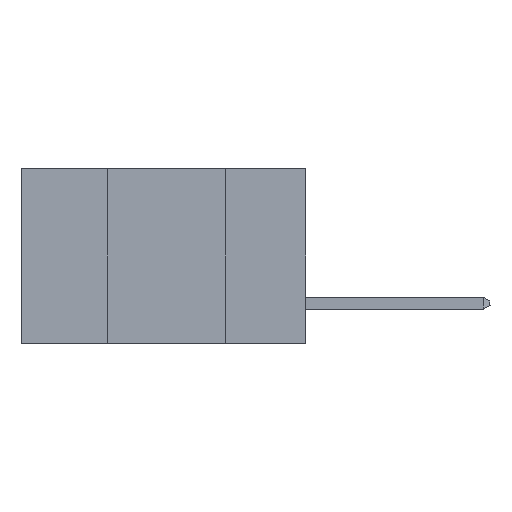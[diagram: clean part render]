
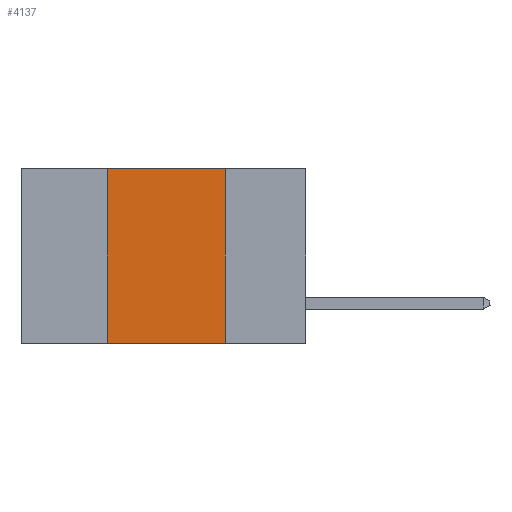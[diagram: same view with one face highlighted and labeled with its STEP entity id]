
A CAD part, left-side view. The second image highlights one B-rep face of the part: STEP entity #4137.
In plain terms, the highlighted planar face has unit normal (-1, 0, 0).
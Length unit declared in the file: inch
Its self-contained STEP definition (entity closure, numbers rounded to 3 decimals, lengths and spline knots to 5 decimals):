
#269 = VERTEX_POINT ( 'NONE', #7787 ) ;
#342 = LINE ( 'NONE', #3607, #6669 ) ;
#1699 = ORIENTED_EDGE ( 'NONE', *, *, #10057, .F. ) ;
#2125 = AXIS2_PLACEMENT_3D ( 'NONE', #2295, #12013, #2155 ) ;
#2155 = DIRECTION ( 'NONE',  ( 0., 0., -1. ) ) ;
#2295 = CARTESIAN_POINT ( 'NONE',  ( 0., 0.6, 0. ) ) ;
#2919 = VECTOR ( 'NONE', #16156, 39.37008 ) ;
#3607 = CARTESIAN_POINT ( 'NONE',  ( 0., 0.6, -0.37 ) ) ;
#4137 = ADVANCED_FACE ( 'NONE', ( #20505 ), #16693, .F. ) ;
#4682 = LINE ( 'NONE', #4693, #2919 ) ;
#4693 = CARTESIAN_POINT ( 'NONE',  ( 0., 0.42, 0. ) ) ;
#4762 = VERTEX_POINT ( 'NONE', #17588 ) ;
#5704 = LINE ( 'NONE', #12455, #12266 ) ;
#5730 = ORIENTED_EDGE ( 'NONE', *, *, #14791, .F. ) ;
#6284 = ORIENTED_EDGE ( 'NONE', *, *, #8999, .F. ) ;
#6669 = VECTOR ( 'NONE', #9724, 39.37008 ) ;
#6997 = LINE ( 'NONE', #11406, #18600 ) ;
#7319 = VERTEX_POINT ( 'NONE', #19278 ) ;
#7787 = CARTESIAN_POINT ( 'NONE',  ( 0., 0.42, 0. ) ) ;
#8999 = EDGE_CURVE ( 'NONE', #9350, #4762, #6997, .T. ) ;
#9350 = VERTEX_POINT ( 'NONE', #15763 ) ;
#9724 = DIRECTION ( 'NONE',  ( 0., -1., 0. ) ) ;
#10057 = EDGE_CURVE ( 'NONE', #7319, #269, #4682, .T. ) ;
#10833 = EDGE_LOOP ( 'NONE', ( #6284, #5730, #1699, #12903 ) ) ;
#11406 = CARTESIAN_POINT ( 'NONE',  ( 0., 0.17, 0. ) ) ;
#12013 = DIRECTION ( 'NONE',  ( 1., 0., 0. ) ) ;
#12266 = VECTOR ( 'NONE', #17042, 39.37008 ) ;
#12455 = CARTESIAN_POINT ( 'NONE',  ( 0., 0.6, 0. ) ) ;
#12903 = ORIENTED_EDGE ( 'NONE', *, *, #13104, .T. ) ;
#13104 = EDGE_CURVE ( 'NONE', #7319, #4762, #342, .T. ) ;
#14791 = EDGE_CURVE ( 'NONE', #269, #9350, #5704, .T. ) ;
#15763 = CARTESIAN_POINT ( 'NONE',  ( 0., 0.17, 0. ) ) ;
#16156 = DIRECTION ( 'NONE',  ( 0., 0., 1. ) ) ;
#16693 = PLANE ( 'NONE',  #2125 ) ;
#17042 = DIRECTION ( 'NONE',  ( 0., -1., 0. ) ) ;
#17588 = CARTESIAN_POINT ( 'NONE',  ( 0., 0.17, -0.37 ) ) ;
#18600 = VECTOR ( 'NONE', #19571, 39.37008 ) ;
#19278 = CARTESIAN_POINT ( 'NONE',  ( 0., 0.42, -0.37 ) ) ;
#19571 = DIRECTION ( 'NONE',  ( 0., 0., -1. ) ) ;
#20505 = FACE_OUTER_BOUND ( 'NONE', #10833, .T. ) ;
